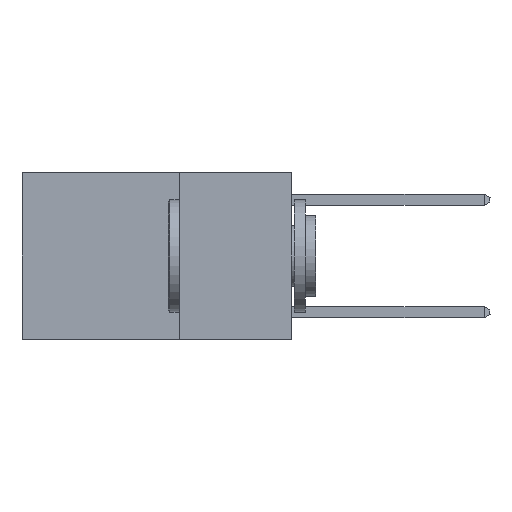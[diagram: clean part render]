
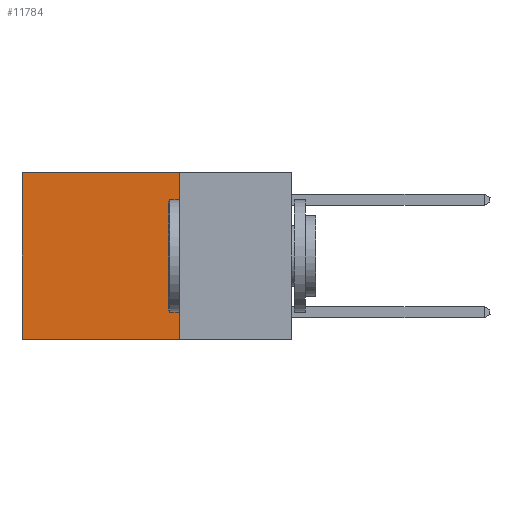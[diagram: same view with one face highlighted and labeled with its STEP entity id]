
A CAD part, left-side view. The second image highlights one B-rep face of the part: STEP entity #11784.
In plain terms, the highlighted planar face has unit normal (-1, 0, 0).
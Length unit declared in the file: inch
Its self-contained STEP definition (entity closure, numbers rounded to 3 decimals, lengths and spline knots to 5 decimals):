
#144 = EDGE_LOOP ( 'NONE', ( #4832, #2038, #5800, #481 ) ) ;
#481 = ORIENTED_EDGE ( 'NONE', *, *, #6470, .T. ) ;
#1263 = CARTESIAN_POINT ( 'NONE',  ( 0.2625, 0.25, 0. ) ) ;
#1972 = VERTEX_POINT ( 'NONE', #22704 ) ;
#2038 = ORIENTED_EDGE ( 'NONE', *, *, #5549, .F. ) ;
#2623 = VECTOR ( 'NONE', #9821, 39.37008 ) ;
#4832 = ORIENTED_EDGE ( 'NONE', *, *, #18817, .T. ) ;
#5549 = EDGE_CURVE ( 'NONE', #17749, #10744, #22410, .T. ) ;
#5800 = ORIENTED_EDGE ( 'NONE', *, *, #11441, .F. ) ;
#6470 = EDGE_CURVE ( 'NONE', #7059, #1972, #7989, .T. ) ;
#7018 = DIRECTION ( 'NONE',  ( 1., 0., 0. ) ) ;
#7059 = VERTEX_POINT ( 'NONE', #15646 ) ;
#7454 = AXIS2_PLACEMENT_3D ( 'NONE', #1263, #7018, #14154 ) ;
#7989 = LINE ( 'NONE', #16806, #2623 ) ;
#8750 = LINE ( 'NONE', #21924, #17683 ) ;
#9475 = DIRECTION ( 'NONE',  ( 0., 1., 0. ) ) ;
#9821 = DIRECTION ( 'NONE',  ( 0., 1., 0. ) ) ;
#10098 = VECTOR ( 'NONE', #14058, 39.37008 ) ;
#10312 = CARTESIAN_POINT ( 'NONE',  ( 0.2625, 0.6, 0. ) ) ;
#10744 = VERTEX_POINT ( 'NONE', #11609 ) ;
#10766 = FACE_OUTER_BOUND ( 'NONE', #144, .T. ) ;
#11441 = EDGE_CURVE ( 'NONE', #7059, #17749, #8750, .T. ) ;
#11609 = CARTESIAN_POINT ( 'NONE',  ( 0.2625, 0.6, -0.37 ) ) ;
#11784 = ADVANCED_FACE ( 'NONE', ( #10766 ), #17768, .F. ) ;
#14058 = DIRECTION ( 'NONE',  ( 0., 0., -1. ) ) ;
#14154 = DIRECTION ( 'NONE',  ( 0., 0., -1. ) ) ;
#15646 = CARTESIAN_POINT ( 'NONE',  ( 0.2625, 0.25, 0. ) ) ;
#16806 = CARTESIAN_POINT ( 'NONE',  ( 0.2625, 0.25, 0. ) ) ;
#17324 = LINE ( 'NONE', #10312, #10098 ) ;
#17683 = VECTOR ( 'NONE', #23751, 39.37008 ) ;
#17749 = VERTEX_POINT ( 'NONE', #17809 ) ;
#17768 = PLANE ( 'NONE',  #7454 ) ;
#17809 = CARTESIAN_POINT ( 'NONE',  ( 0.2625, 0.25, -0.37 ) ) ;
#18817 = EDGE_CURVE ( 'NONE', #1972, #10744, #17324, .T. ) ;
#18986 = CARTESIAN_POINT ( 'NONE',  ( 0.2625, 0.25, -0.37 ) ) ;
#20322 = VECTOR ( 'NONE', #9475, 39.37008 ) ;
#21924 = CARTESIAN_POINT ( 'NONE',  ( 0.2625, 0.25, 0. ) ) ;
#22410 = LINE ( 'NONE', #18986, #20322 ) ;
#22704 = CARTESIAN_POINT ( 'NONE',  ( 0.2625, 0.6, 0. ) ) ;
#23751 = DIRECTION ( 'NONE',  ( 0., 0., -1. ) ) ;
